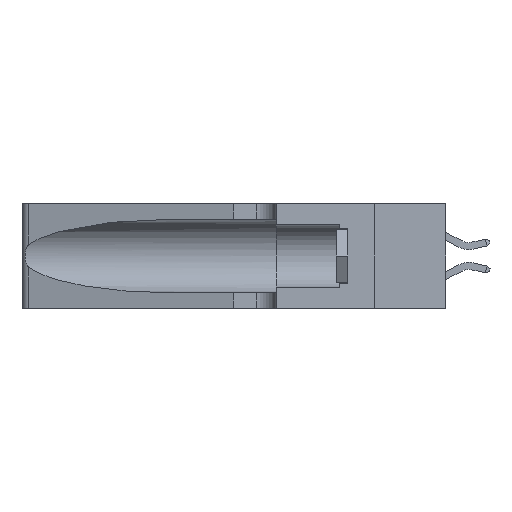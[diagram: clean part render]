
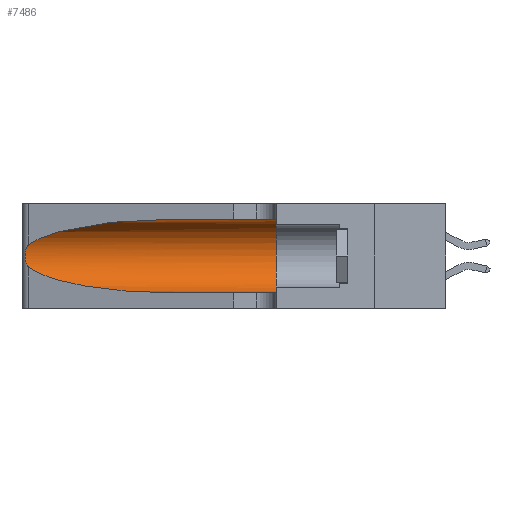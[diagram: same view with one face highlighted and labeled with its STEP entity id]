
A CAD part, left-side view. The second image highlights one B-rep face of the part: STEP entity #7486.
In plain terms, the highlighted cylindrical face has radius 3.308 mm (diameter 6.617 mm), a partial arc.
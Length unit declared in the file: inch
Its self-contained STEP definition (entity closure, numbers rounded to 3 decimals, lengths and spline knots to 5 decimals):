
#38 = VERTEX_POINT ( 'NONE', #10304 ) ;
#62 = CARTESIAN_POINT ( 'NONE',  ( 0.18966, 0.96281, 0.05475 ) ) ;
#67 = VERTEX_POINT ( 'NONE', #18112 ) ;
#146 = CARTESIAN_POINT ( 'NONE',  ( 0.25487, 1.22718, 0.14631 ) ) ;
#660 = B_SPLINE_CURVE_WITH_KNOTS ( 'NONE', 3,
 ( #12922, #3141, #14568, #4831, #16180, #6466, #17805, #8111, #19386, #9776, #20965, #11397, #1545, #12998 ),
 .UNSPECIFIED., .F., .F.,
 ( 4, 2, 2, 2, 2, 2, 4 ),
 ( 0., 0.00027, 0.00053, 0.00107, 0.0016, 0.00187, 0.00214 ),
 .UNSPECIFIED. ) ;
#1062 =( BOUNDED_CURVE ( )  B_SPLINE_CURVE ( 3, ( #6665, #16390, #62, #11599 ),
 .UNSPECIFIED., .F., .F. ) 
 B_SPLINE_CURVE_WITH_KNOTS ( ( 4, 4 ),
 ( 3.44316, 4.71239 ),
 .UNSPECIFIED. ) 
 CURVE ( )  GEOMETRIC_REPRESENTATION_ITEM ( )  RATIONAL_B_SPLINE_CURVE ( ( 1., 0.87, 0.87, 1. ) ) 
 REPRESENTATION_ITEM ( '' )  );
#1467 =( BOUNDED_CURVE ( )  B_SPLINE_CURVE ( 3, ( #6583, #4965, #14679, #8240 ),
 .UNSPECIFIED., .F., .T. ) 
 B_SPLINE_CURVE_WITH_KNOTS ( ( 4, 4 ),
 ( 1.5708, 2.84003 ),
 .UNSPECIFIED. ) 
 CURVE ( )  GEOMETRIC_REPRESENTATION_ITEM ( )  RATIONAL_B_SPLINE_CURVE ( ( 1., 0.87, 0.87, 1. ) ) 
 REPRESENTATION_ITEM ( '' )  );
#1545 = CARTESIAN_POINT ( 'NONE',  ( 0.25555, 1.22993, 0.14849 ) ) ;
#1719 = CARTESIAN_POINT ( 'NONE',  ( 0.25487, 1.22718, 0.22369 ) ) ;
#1943 = ORIENTED_EDGE ( 'NONE', *, *, #5498, .F. ) ;
#2714 = ORIENTED_EDGE ( 'NONE', *, *, #3629, .T. ) ;
#3141 = CARTESIAN_POINT ( 'NONE',  ( 0.25555, 1.22994, 0.2215 ) ) ;
#3407 = AXIS2_PLACEMENT_3D ( 'NONE', #6839, #18161, #8512 ) ;
#3563 = AXIS2_PLACEMENT_3D ( 'NONE', #13811, #7324, #9007 ) ;
#3629 = EDGE_CURVE ( 'NONE', #17020, #5445, #1467, .T. ) ;
#4077 = LINE ( 'NONE', #15488, #8459 ) ;
#4831 = CARTESIAN_POINT ( 'NONE',  ( 0.25787, 1.23484, 0.2124 ) ) ;
#4965 = CARTESIAN_POINT ( 'NONE',  ( 0.18966, 0.96281, 0.31525 ) ) ;
#5445 = VERTEX_POINT ( 'NONE', #1719 ) ;
#5498 = EDGE_CURVE ( 'NONE', #67, #6555, #16911, .T. ) ;
#5896 = FACE_OUTER_BOUND ( 'NONE', #19242, .T. ) ;
#6466 = CARTESIAN_POINT ( 'NONE',  ( 0.26018, 1.23835, 0.19895 ) ) ;
#6555 = VERTEX_POINT ( 'NONE', #8092 ) ;
#6583 = CARTESIAN_POINT ( 'NONE',  ( 0.1305, 0.72297, 0.31525 ) ) ;
#6665 = CARTESIAN_POINT ( 'NONE',  ( 0.25487, 1.22718, 0.14631 ) ) ;
#6839 = CARTESIAN_POINT ( 'NONE',  ( 0.1305, 0.35, 0.185 ) ) ;
#6879 = CARTESIAN_POINT ( 'NONE',  ( 0.1305, 0.72297, 0.31525 ) ) ;
#7324 = DIRECTION ( 'NONE',  ( 0., -1., 0. ) ) ;
#7486 = ADVANCED_FACE ( 'NONE', ( #5896 ), #9224, .F. ) ;
#7813 = EDGE_CURVE ( 'NONE', #5445, #15230, #660, .T. ) ;
#8092 = CARTESIAN_POINT ( 'NONE',  ( 0.1305, 0.35, 0.05475 ) ) ;
#8111 = CARTESIAN_POINT ( 'NONE',  ( 0.26075, 1.23896, 0.178 ) ) ;
#8240 = CARTESIAN_POINT ( 'NONE',  ( 0.25487, 1.22718, 0.22369 ) ) ;
#8459 = VECTOR ( 'NONE', #13931, 39.37008 ) ;
#8512 = DIRECTION ( 'NONE',  ( 0., 0., 1. ) ) ;
#8961 = ORIENTED_EDGE ( 'NONE', *, *, #7813, .T. ) ;
#9007 = DIRECTION ( 'NONE',  ( 0., 0., -1. ) ) ;
#9224 = CYLINDRICAL_SURFACE ( 'NONE', #3563, 0.13025 ) ;
#9776 = CARTESIAN_POINT ( 'NONE',  ( 0.25856, 1.23593, 0.16098 ) ) ;
#9786 = EDGE_CURVE ( 'NONE', #38, #6555, #13193, .T. ) ;
#10304 = CARTESIAN_POINT ( 'NONE',  ( 0.1305, 0.72297, 0.05475 ) ) ;
#11397 = CARTESIAN_POINT ( 'NONE',  ( 0.25639, 1.23186, 0.15144 ) ) ;
#11599 = CARTESIAN_POINT ( 'NONE',  ( 0.1305, 0.72297, 0.05475 ) ) ;
#11879 = DIRECTION ( 'NONE',  ( 0., -1., 0. ) ) ;
#12922 = CARTESIAN_POINT ( 'NONE',  ( 0.25487, 1.22718, 0.22369 ) ) ;
#12998 = CARTESIAN_POINT ( 'NONE',  ( 0.25487, 1.22718, 0.14631 ) ) ;
#13193 = LINE ( 'NONE', #15096, #17481 ) ;
#13811 = CARTESIAN_POINT ( 'NONE',  ( 0.1305, 1.61858, 0.185 ) ) ;
#13931 = DIRECTION ( 'NONE',  ( 0., -1., 0. ) ) ;
#14568 = CARTESIAN_POINT ( 'NONE',  ( 0.25639, 1.23184, 0.21858 ) ) ;
#14679 = CARTESIAN_POINT ( 'NONE',  ( 0.2373, 1.15595, 0.28018 ) ) ;
#15096 = CARTESIAN_POINT ( 'NONE',  ( 0.1305, 1.61858, 0.05475 ) ) ;
#15230 = VERTEX_POINT ( 'NONE', #146 ) ;
#15488 = CARTESIAN_POINT ( 'NONE',  ( 0.1305, 1.61858, 0.31525 ) ) ;
#16046 = ORIENTED_EDGE ( 'NONE', *, *, #9786, .T. ) ;
#16180 = CARTESIAN_POINT ( 'NONE',  ( 0.25854, 1.2359, 0.20912 ) ) ;
#16390 = CARTESIAN_POINT ( 'NONE',  ( 0.2373, 1.15595, 0.08982 ) ) ;
#16845 = EDGE_CURVE ( 'NONE', #17020, #67, #4077, .T. ) ;
#16911 = CIRCLE ( 'NONE', #3407, 0.13025 ) ;
#17020 = VERTEX_POINT ( 'NONE', #6879 ) ;
#17481 = VECTOR ( 'NONE', #11879, 39.37008 ) ;
#17805 = CARTESIAN_POINT ( 'NONE',  ( 0.26075, 1.23896, 0.19203 ) ) ;
#18112 = CARTESIAN_POINT ( 'NONE',  ( 0.1305, 0.35, 0.31525 ) ) ;
#18161 = DIRECTION ( 'NONE',  ( 0., 1., 0. ) ) ;
#19242 = EDGE_LOOP ( 'NONE', ( #2714, #8961, #20685, #16046, #1943, #20537 ) ) ;
#19386 = CARTESIAN_POINT ( 'NONE',  ( 0.26017, 1.23833, 0.17102 ) ) ;
#20537 = ORIENTED_EDGE ( 'NONE', *, *, #16845, .F. ) ;
#20685 = ORIENTED_EDGE ( 'NONE', *, *, #20999, .T. ) ;
#20965 = CARTESIAN_POINT ( 'NONE',  ( 0.25789, 1.23486, 0.15765 ) ) ;
#20999 = EDGE_CURVE ( 'NONE', #15230, #38, #1062, .T. ) ;
